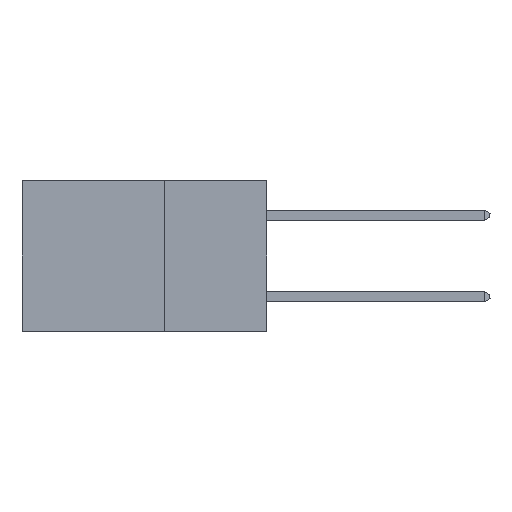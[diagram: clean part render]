
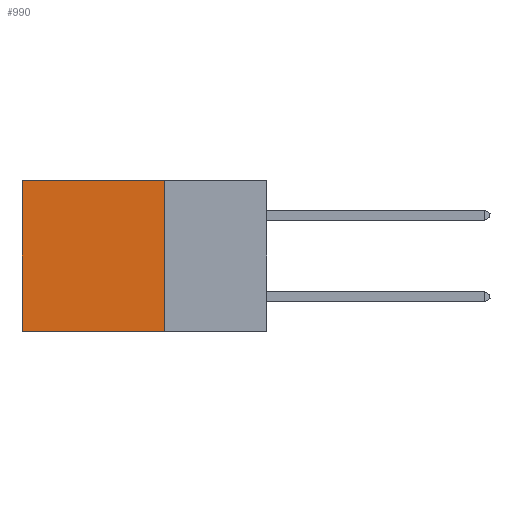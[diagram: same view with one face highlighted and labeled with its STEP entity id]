
A CAD part, left-side view. The second image highlights one B-rep face of the part: STEP entity #990.
In plain terms, the highlighted planar face has unit normal (-1, 0, 0).
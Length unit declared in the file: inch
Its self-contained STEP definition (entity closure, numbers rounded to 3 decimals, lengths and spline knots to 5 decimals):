
#990 = ADVANCED_FACE ( 'NONE', ( #2832 ), #3509, .F. ) ;
#1591 = CARTESIAN_POINT ( 'NONE',  ( 0.2875, 0.25, 0. ) ) ;
#1889 = LINE ( 'NONE', #15534, #7893 ) ;
#1899 = CARTESIAN_POINT ( 'NONE',  ( 0.2875, 0.25, -0.37 ) ) ;
#1974 = VERTEX_POINT ( 'NONE', #1591 ) ;
#2832 = FACE_OUTER_BOUND ( 'NONE', #15976, .T. ) ;
#3509 = PLANE ( 'NONE',  #15426 ) ;
#3961 = DIRECTION ( 'NONE',  ( 0., 1., 0. ) ) ;
#5019 = CARTESIAN_POINT ( 'NONE',  ( 0.2875, 0.25, 0. ) ) ;
#5608 = VECTOR ( 'NONE', #3961, 39.37008 ) ;
#6770 = VERTEX_POINT ( 'NONE', #1899 ) ;
#6775 = CARTESIAN_POINT ( 'NONE',  ( 0.2875, 0.25, -0.37 ) ) ;
#7083 = CARTESIAN_POINT ( 'NONE',  ( 0.2875, 0.25, 0. ) ) ;
#7892 = EDGE_CURVE ( 'NONE', #8055, #20750, #1889, .T. ) ;
#7893 = VECTOR ( 'NONE', #15698, 39.37008 ) ;
#8055 = VERTEX_POINT ( 'NONE', #23655 ) ;
#9186 = VECTOR ( 'NONE', #21512, 39.37008 ) ;
#9587 = ORIENTED_EDGE ( 'NONE', *, *, #7892, .T. ) ;
#10511 = LINE ( 'NONE', #6775, #19681 ) ;
#10691 = DIRECTION ( 'NONE',  ( 0., 1., 0. ) ) ;
#12823 = ORIENTED_EDGE ( 'NONE', *, *, #14139, .F. ) ;
#12827 = ORIENTED_EDGE ( 'NONE', *, *, #22204, .F. ) ;
#14139 = EDGE_CURVE ( 'NONE', #6770, #20750, #10511, .T. ) ;
#15426 = AXIS2_PLACEMENT_3D ( 'NONE', #5019, #21618, #19759 ) ;
#15534 = CARTESIAN_POINT ( 'NONE',  ( 0.2875, 0.6, 0. ) ) ;
#15698 = DIRECTION ( 'NONE',  ( 0., 0., -1. ) ) ;
#15976 = EDGE_LOOP ( 'NONE', ( #9587, #12823, #12827, #22948 ) ) ;
#17146 = CARTESIAN_POINT ( 'NONE',  ( 0.2875, 0.6, -0.37 ) ) ;
#18424 = CARTESIAN_POINT ( 'NONE',  ( 0.2875, 0.25, 0. ) ) ;
#19151 = EDGE_CURVE ( 'NONE', #1974, #8055, #21394, .T. ) ;
#19681 = VECTOR ( 'NONE', #10691, 39.37008 ) ;
#19759 = DIRECTION ( 'NONE',  ( 0., 0., -1. ) ) ;
#20750 = VERTEX_POINT ( 'NONE', #17146 ) ;
#21263 = LINE ( 'NONE', #7083, #9186 ) ;
#21394 = LINE ( 'NONE', #18424, #5608 ) ;
#21512 = DIRECTION ( 'NONE',  ( 0., 0., -1. ) ) ;
#21618 = DIRECTION ( 'NONE',  ( 1., 0., 0. ) ) ;
#22204 = EDGE_CURVE ( 'NONE', #1974, #6770, #21263, .T. ) ;
#22948 = ORIENTED_EDGE ( 'NONE', *, *, #19151, .T. ) ;
#23655 = CARTESIAN_POINT ( 'NONE',  ( 0.2875, 0.6, 0. ) ) ;
